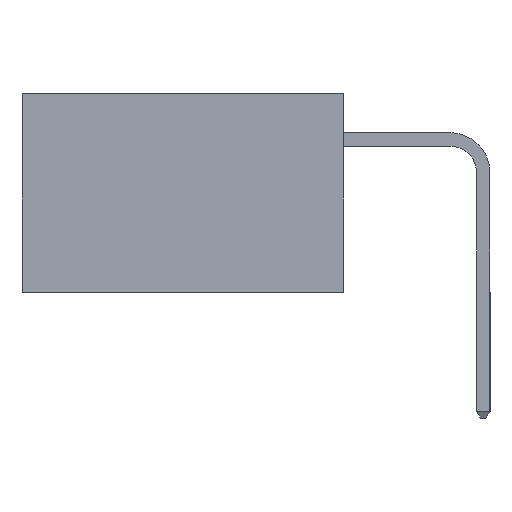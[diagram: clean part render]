
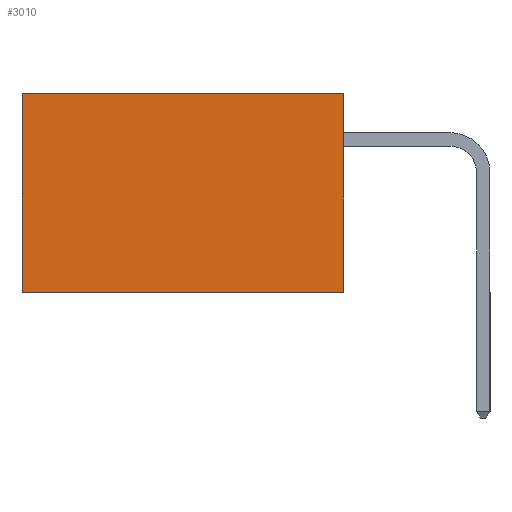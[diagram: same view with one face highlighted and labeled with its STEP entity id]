
A CAD part, left-side view. The second image highlights one B-rep face of the part: STEP entity #3010.
In plain terms, the highlighted planar face has unit normal (-1, 0, 0).
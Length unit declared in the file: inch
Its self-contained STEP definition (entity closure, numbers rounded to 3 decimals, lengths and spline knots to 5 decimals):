
#458 = ORIENTED_EDGE ( 'NONE', *, *, #4427, .T. ) ;
#1266 = CARTESIAN_POINT ( 'NONE',  ( 0.298, 0., -0.37 ) ) ;
#1828 = CARTESIAN_POINT ( 'NONE',  ( 0.298, 0.6, -0.37 ) ) ;
#2527 = CARTESIAN_POINT ( 'NONE',  ( 0.298, 0., 0. ) ) ;
#3010 = ADVANCED_FACE ( 'NONE', ( #13035 ), #15581, .F. ) ;
#3585 = VERTEX_POINT ( 'NONE', #7548 ) ;
#3586 = DIRECTION ( 'NONE',  ( 0., 0., -1. ) ) ;
#4427 = EDGE_CURVE ( 'NONE', #16623, #3585, #10321, .T. ) ;
#4682 = EDGE_CURVE ( 'NONE', #19951, #11816, #14481, .T. ) ;
#5795 = VECTOR ( 'NONE', #7357, 39.37008 ) ;
#6568 = LINE ( 'NONE', #10404, #18879 ) ;
#7357 = DIRECTION ( 'NONE',  ( 0., 1., 0. ) ) ;
#7381 = CARTESIAN_POINT ( 'NONE',  ( 0.298, 0., 0. ) ) ;
#7398 = VECTOR ( 'NONE', #11387, 39.37008 ) ;
#7548 = CARTESIAN_POINT ( 'NONE',  ( 0.298, 0.6, 0. ) ) ;
#7567 = EDGE_CURVE ( 'NONE', #16623, #19951, #16344, .T. ) ;
#8394 = CARTESIAN_POINT ( 'NONE',  ( 0.298, 0., 0. ) ) ;
#10013 = ORIENTED_EDGE ( 'NONE', *, *, #19087, .T. ) ;
#10321 = LINE ( 'NONE', #7381, #5795 ) ;
#10404 = CARTESIAN_POINT ( 'NONE',  ( 0.298, 0.6, 0. ) ) ;
#10657 = CARTESIAN_POINT ( 'NONE',  ( 0.298, 0., 0. ) ) ;
#11387 = DIRECTION ( 'NONE',  ( 0., 0., -1. ) ) ;
#11816 = VERTEX_POINT ( 'NONE', #1828 ) ;
#12097 = DIRECTION ( 'NONE',  ( 0., 1., 0. ) ) ;
#13035 = FACE_OUTER_BOUND ( 'NONE', #20820, .T. ) ;
#13409 = DIRECTION ( 'NONE',  ( 0., 0., -1. ) ) ;
#13435 = DIRECTION ( 'NONE',  ( 1., 0., 0. ) ) ;
#14481 = LINE ( 'NONE', #1266, #18384 ) ;
#15581 = PLANE ( 'NONE',  #16674 ) ;
#16344 = LINE ( 'NONE', #10657, #7398 ) ;
#16623 = VERTEX_POINT ( 'NONE', #8394 ) ;
#16674 = AXIS2_PLACEMENT_3D ( 'NONE', #2527, #13435, #13409 ) ;
#17819 = ORIENTED_EDGE ( 'NONE', *, *, #4682, .F. ) ;
#18384 = VECTOR ( 'NONE', #12097, 39.37008 ) ;
#18879 = VECTOR ( 'NONE', #3586, 39.37008 ) ;
#19053 = ORIENTED_EDGE ( 'NONE', *, *, #7567, .F. ) ;
#19087 = EDGE_CURVE ( 'NONE', #3585, #11816, #6568, .T. ) ;
#19332 = CARTESIAN_POINT ( 'NONE',  ( 0.298, 0., -0.37 ) ) ;
#19951 = VERTEX_POINT ( 'NONE', #19332 ) ;
#20820 = EDGE_LOOP ( 'NONE', ( #10013, #17819, #19053, #458 ) ) ;
